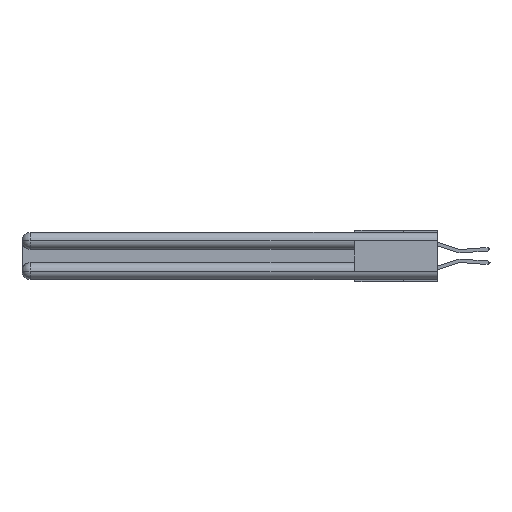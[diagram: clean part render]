
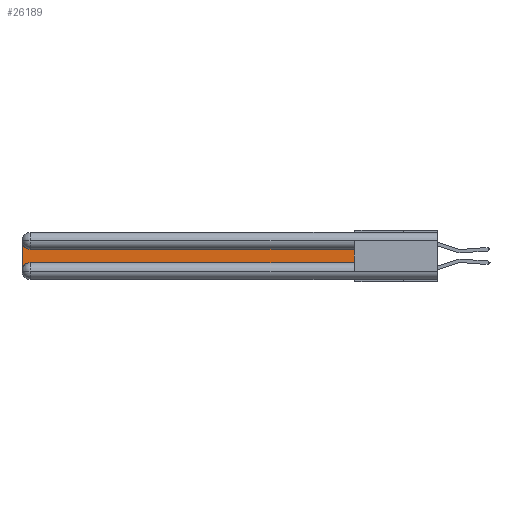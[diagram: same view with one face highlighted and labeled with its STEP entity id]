
A CAD part, left-side view. The second image highlights one B-rep face of the part: STEP entity #26189.
In plain terms, the highlighted planar face has unit normal (-1, 0, 0).
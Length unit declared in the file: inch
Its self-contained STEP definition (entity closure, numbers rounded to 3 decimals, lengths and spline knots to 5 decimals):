
#813 = CARTESIAN_POINT ( 'NONE',  ( 0.075, 3., -0.0625 ) ) ;
#1281 = EDGE_CURVE ( 'NONE', #24617, #5204, #20008, .T. ) ;
#1595 = CARTESIAN_POINT ( 'NONE',  ( 0.075, 3., -0.2775 ) ) ;
#2070 = VERTEX_POINT ( 'NONE', #1595 ) ;
#2134 = CARTESIAN_POINT ( 'NONE',  ( 0.075, 0.6, -0.1225 ) ) ;
#2164 = DIRECTION ( 'NONE',  ( 0., 0., 1. ) ) ;
#2180 = ORIENTED_EDGE ( 'NONE', *, *, #8865, .T. ) ;
#2302 = DIRECTION ( 'NONE',  ( 1., 0., 0. ) ) ;
#2345 = CARTESIAN_POINT ( 'NONE',  ( 0.075, 0.6, -0.2175 ) ) ;
#2389 = DIRECTION ( 'NONE',  ( 0., 0., -1. ) ) ;
#2559 = AXIS2_PLACEMENT_3D ( 'NONE', #5298, #17939, #13905 ) ;
#2862 = AXIS2_PLACEMENT_3D ( 'NONE', #15595, #25828, #23574 ) ;
#3489 = VECTOR ( 'NONE', #2164, 39.37008 ) ;
#3640 = CARTESIAN_POINT ( 'NONE',  ( 0.075, 2.94, -0.2175 ) ) ;
#4141 = EDGE_CURVE ( 'NONE', #14445, #24617, #25198, .T. ) ;
#4618 = CARTESIAN_POINT ( 'NONE',  ( 0.075, 2.94, -0.1225 ) ) ;
#5204 = VERTEX_POINT ( 'NONE', #21745 ) ;
#5298 = CARTESIAN_POINT ( 'NONE',  ( 0.075, 3., -0.1225 ) ) ;
#5812 = LINE ( 'NONE', #2134, #13274 ) ;
#5920 = VERTEX_POINT ( 'NONE', #4618 ) ;
#6478 = CARTESIAN_POINT ( 'NONE',  ( 0.075, 2.94, -0.2775 ) ) ;
#7137 = AXIS2_PLACEMENT_3D ( 'NONE', #6478, #2302, #2389 ) ;
#7962 = CARTESIAN_POINT ( 'NONE',  ( 0.075, 0.6, -0.2175 ) ) ;
#8865 = EDGE_CURVE ( 'NONE', #2070, #14445, #18050, .T. ) ;
#10413 = VERTEX_POINT ( 'NONE', #813 ) ;
#11375 = ORIENTED_EDGE ( 'NONE', *, *, #18398, .T. ) ;
#11901 = CIRCLE ( 'NONE', #2862, 0.06 ) ;
#12273 = ORIENTED_EDGE ( 'NONE', *, *, #12768, .T. ) ;
#12428 = ORIENTED_EDGE ( 'NONE', *, *, #20887, .T. ) ;
#12768 = EDGE_CURVE ( 'NONE', #5920, #10413, #11901, .T. ) ;
#13274 = VECTOR ( 'NONE', #23090, 39.37008 ) ;
#13905 = DIRECTION ( 'NONE',  ( 0., 0., -1. ) ) ;
#14054 = EDGE_LOOP ( 'NONE', ( #12428, #12273, #11375, #2180, #23041, #19879 ) ) ;
#14445 = VERTEX_POINT ( 'NONE', #3640 ) ;
#15388 = VECTOR ( 'NONE', #18990, 39.37008 ) ;
#15595 = CARTESIAN_POINT ( 'NONE',  ( 0.075, 2.94, -0.0625 ) ) ;
#17939 = DIRECTION ( 'NONE',  ( 1., 0., 0. ) ) ;
#18050 = CIRCLE ( 'NONE', #7137, 0.06 ) ;
#18398 = EDGE_CURVE ( 'NONE', #10413, #2070, #18663, .T. ) ;
#18663 = LINE ( 'NONE', #18724, #15388 ) ;
#18724 = CARTESIAN_POINT ( 'NONE',  ( 0.075, 3., -0.2175 ) ) ;
#18990 = DIRECTION ( 'NONE',  ( 0., 0., -1. ) ) ;
#19879 = ORIENTED_EDGE ( 'NONE', *, *, #1281, .T. ) ;
#20008 = LINE ( 'NONE', #2345, #3489 ) ;
#20887 = EDGE_CURVE ( 'NONE', #5204, #5920, #5812, .T. ) ;
#21745 = CARTESIAN_POINT ( 'NONE',  ( 0.075, 0.6, -0.1225 ) ) ;
#22754 = DIRECTION ( 'NONE',  ( 0., -1., 0. ) ) ;
#22929 = VECTOR ( 'NONE', #22754, 39.37008 ) ;
#23024 = FACE_OUTER_BOUND ( 'NONE', #14054, .T. ) ;
#23041 = ORIENTED_EDGE ( 'NONE', *, *, #4141, .T. ) ;
#23090 = DIRECTION ( 'NONE',  ( 0., 1., 0. ) ) ;
#23574 = DIRECTION ( 'NONE',  ( 0., 0., -1. ) ) ;
#23669 = CARTESIAN_POINT ( 'NONE',  ( 0.075, 0.6, -0.2175 ) ) ;
#24617 = VERTEX_POINT ( 'NONE', #23669 ) ;
#25198 = LINE ( 'NONE', #7962, #22929 ) ;
#25310 = PLANE ( 'NONE',  #2559 ) ;
#25828 = DIRECTION ( 'NONE',  ( 1., 0., 0. ) ) ;
#26189 = ADVANCED_FACE ( 'NONE', ( #23024 ), #25310, .F. ) ;
